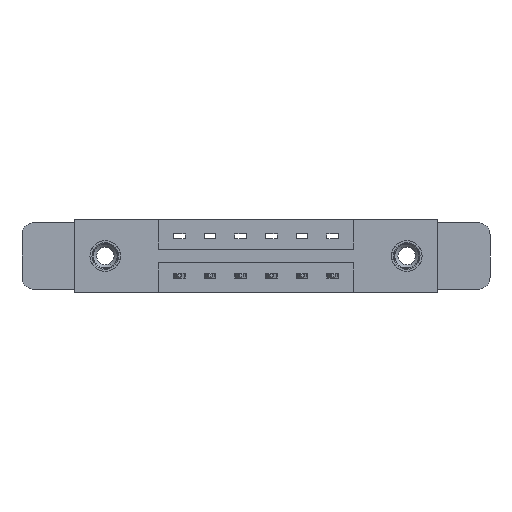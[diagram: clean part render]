
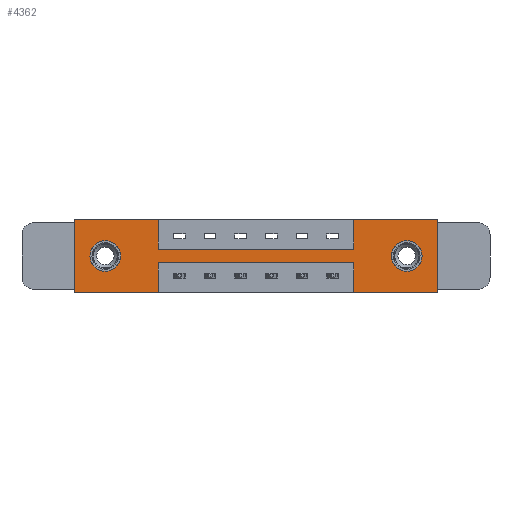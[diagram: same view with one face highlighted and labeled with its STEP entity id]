
A CAD part, front view. The second image highlights one B-rep face of the part: STEP entity #4362.
In plain terms, the highlighted planar face has unit normal (0, -1, 0).
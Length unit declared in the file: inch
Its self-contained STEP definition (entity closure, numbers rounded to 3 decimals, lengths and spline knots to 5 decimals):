
#9 = EDGE_LOOP ( 'NONE', ( #1963, #6554 ) ) ;
#53 = DIRECTION ( 'NONE',  ( 0., 1., 0. ) ) ;
#268 = VECTOR ( 'NONE', #10527, 39.37008 ) ;
#271 = VERTEX_POINT ( 'NONE', #1004 ) ;
#307 = DIRECTION ( 'NONE',  ( 0., 1., 0. ) ) ;
#468 = CARTESIAN_POINT ( 'NONE',  ( 0., 0., 0. ) ) ;
#487 = LINE ( 'NONE', #468, #2744 ) ;
#525 = CARTESIAN_POINT ( 'NONE',  ( 1.417, 0., -0.22 ) ) ;
#589 = DIRECTION ( 'NONE',  ( 0., -1., 0. ) ) ;
#739 = ORIENTED_EDGE ( 'NONE', *, *, #3154, .T. ) ;
#833 = EDGE_CURVE ( 'NONE', #2236, #11252, #10654, .T. ) ;
#843 = VERTEX_POINT ( 'NONE', #4582 ) ;
#922 = EDGE_CURVE ( 'NONE', #6024, #10262, #3065, .T. ) ;
#923 = VERTEX_POINT ( 'NONE', #1843 ) ;
#1004 = CARTESIAN_POINT ( 'NONE',  ( 0.425, 0., -0.15 ) ) ;
#1042 = CARTESIAN_POINT ( 'NONE',  ( 0.155, 0., -0.185 ) ) ;
#1116 = EDGE_CURVE ( 'NONE', #10430, #5213, #7602, .T. ) ;
#1382 = CARTESIAN_POINT ( 'NONE',  ( 0.425, 0., 0. ) ) ;
#1463 = LINE ( 'NONE', #9591, #10608 ) ;
#1606 = CARTESIAN_POINT ( 'NONE',  ( 0., 0., 0. ) ) ;
#1753 = CARTESIAN_POINT ( 'NONE',  ( 0., 0., -0.37 ) ) ;
#1778 = ORIENTED_EDGE ( 'NONE', *, *, #9428, .F. ) ;
#1800 = EDGE_CURVE ( 'NONE', #6470, #8813, #2345, .T. ) ;
#1843 = CARTESIAN_POINT ( 'NONE',  ( 0., 0., 0. ) ) ;
#1890 = EDGE_CURVE ( 'NONE', #10592, #6024, #8596, .T. ) ;
#1942 = DIRECTION ( 'NONE',  ( 0., 1., 0. ) ) ;
#1943 = DIRECTION ( 'NONE',  ( -1., 0., 0. ) ) ;
#1963 = ORIENTED_EDGE ( 'NONE', *, *, #833, .T. ) ;
#2064 = EDGE_LOOP ( 'NONE', ( #2796, #8260, #10268, #7159, #7033, #7247, #11724, #1778, #2246, #2922, #5707, #10975 ) ) ;
#2178 = CARTESIAN_POINT ( 'NONE',  ( 1.417, 0., 0. ) ) ;
#2236 = VERTEX_POINT ( 'NONE', #5588 ) ;
#2246 = ORIENTED_EDGE ( 'NONE', *, *, #11702, .F. ) ;
#2331 = CARTESIAN_POINT ( 'NONE',  ( 0., 0., -0.37 ) ) ;
#2345 = LINE ( 'NONE', #6467, #4595 ) ;
#2382 = LINE ( 'NONE', #1382, #268 ) ;
#2586 = EDGE_CURVE ( 'NONE', #10262, #6470, #1463, .T. ) ;
#2744 = VECTOR ( 'NONE', #6801, 39.37008 ) ;
#2754 = FACE_BOUND ( 'NONE', #9518, .T. ) ;
#2796 = ORIENTED_EDGE ( 'NONE', *, *, #2586, .F. ) ;
#2803 = CARTESIAN_POINT ( 'NONE',  ( 0.425, 0., -0.22 ) ) ;
#2817 = VECTOR ( 'NONE', #6248, 39.37008 ) ;
#2922 = ORIENTED_EDGE ( 'NONE', *, *, #11115, .F. ) ;
#3005 = VERTEX_POINT ( 'NONE', #10328 ) ;
#3065 = LINE ( 'NONE', #9972, #4051 ) ;
#3154 = EDGE_CURVE ( 'NONE', #843, #7137, #9260, .T. ) ;
#3186 = DIRECTION ( 'NONE',  ( 0., 0., 1. ) ) ;
#3655 = DIRECTION ( 'NONE',  ( 0., 0., 1. ) ) ;
#4051 = VECTOR ( 'NONE', #4507, 39.37008 ) ;
#4255 = LINE ( 'NONE', #5700, #9387 ) ;
#4362 = ADVANCED_FACE ( 'NONE', ( #5420, #2754, #9440 ), #5105, .T. ) ;
#4507 = DIRECTION ( 'NONE',  ( -1., 0., 0. ) ) ;
#4548 = CARTESIAN_POINT ( 'NONE',  ( 1.687, 0., -0.185 ) ) ;
#4582 = CARTESIAN_POINT ( 'NONE',  ( 0.155, 0., -0.107 ) ) ;
#4595 = VECTOR ( 'NONE', #1943, 39.37008 ) ;
#4645 = LINE ( 'NONE', #5330, #2817 ) ;
#4797 = VECTOR ( 'NONE', #9474, 39.37008 ) ;
#4827 = EDGE_CURVE ( 'NONE', #5213, #3005, #487, .T. ) ;
#4835 = DIRECTION ( 'NONE',  ( 0., 0., -1. ) ) ;
#4852 = AXIS2_PLACEMENT_3D ( 'NONE', #5870, #8636, #3186 ) ;
#5105 = PLANE ( 'NONE',  #8727 ) ;
#5134 = DIRECTION ( 'NONE',  ( 0., 0., -1. ) ) ;
#5213 = VERTEX_POINT ( 'NONE', #6055 ) ;
#5268 = AXIS2_PLACEMENT_3D ( 'NONE', #1042, #1942, #3655 ) ;
#5330 = CARTESIAN_POINT ( 'NONE',  ( 0., 0., -0.37 ) ) ;
#5352 = EDGE_CURVE ( 'NONE', #8813, #923, #8725, .T. ) ;
#5420 = FACE_BOUND ( 'NONE', #9, .T. ) ;
#5453 = AXIS2_PLACEMENT_3D ( 'NONE', #4548, #53, #5476 ) ;
#5476 = DIRECTION ( 'NONE',  ( 0., 0., -1. ) ) ;
#5588 = CARTESIAN_POINT ( 'NONE',  ( 1.687, 0., -0.107 ) ) ;
#5700 = CARTESIAN_POINT ( 'NONE',  ( 1.842, 0., 0. ) ) ;
#5707 = ORIENTED_EDGE ( 'NONE', *, *, #5352, .F. ) ;
#5870 = CARTESIAN_POINT ( 'NONE',  ( 0.155, 0., -0.185 ) ) ;
#6024 = VERTEX_POINT ( 'NONE', #525 ) ;
#6029 = CARTESIAN_POINT ( 'NONE',  ( 0.425, 0., 0. ) ) ;
#6055 = CARTESIAN_POINT ( 'NONE',  ( 1.417, 0., 0. ) ) ;
#6162 = VECTOR ( 'NONE', #7579, 39.37008 ) ;
#6248 = DIRECTION ( 'NONE',  ( -1., 0., 0. ) ) ;
#6366 = CARTESIAN_POINT ( 'NONE',  ( 1.417, 0., -0.37 ) ) ;
#6467 = CARTESIAN_POINT ( 'NONE',  ( 0., 0., -0.37 ) ) ;
#6470 = VERTEX_POINT ( 'NONE', #10317 ) ;
#6524 = CIRCLE ( 'NONE', #9713, 0.078 ) ;
#6554 = ORIENTED_EDGE ( 'NONE', *, *, #7571, .T. ) ;
#6642 = DIRECTION ( 'NONE',  ( 0., 0., -1. ) ) ;
#6801 = DIRECTION ( 'NONE',  ( 1., 0., 0. ) ) ;
#7033 = ORIENTED_EDGE ( 'NONE', *, *, #10008, .F. ) ;
#7137 = VERTEX_POINT ( 'NONE', #8942 ) ;
#7159 = ORIENTED_EDGE ( 'NONE', *, *, #8118, .F. ) ;
#7247 = ORIENTED_EDGE ( 'NONE', *, *, #4827, .F. ) ;
#7571 = EDGE_CURVE ( 'NONE', #11252, #2236, #6524, .T. ) ;
#7579 = DIRECTION ( 'NONE',  ( 0., 0., 1. ) ) ;
#7602 = LINE ( 'NONE', #2178, #8315 ) ;
#7781 = VERTEX_POINT ( 'NONE', #7788 ) ;
#7788 = CARTESIAN_POINT ( 'NONE',  ( 1.842, 0., -0.37 ) ) ;
#7966 = DIRECTION ( 'NONE',  ( 0., 0., 1. ) ) ;
#8118 = EDGE_CURVE ( 'NONE', #7781, #10592, #4645, .T. ) ;
#8260 = ORIENTED_EDGE ( 'NONE', *, *, #922, .F. ) ;
#8315 = VECTOR ( 'NONE', #11416, 39.37008 ) ;
#8461 = CARTESIAN_POINT ( 'NONE',  ( 0.425, 0., -0.15 ) ) ;
#8596 = LINE ( 'NONE', #11273, #6162 ) ;
#8601 = CARTESIAN_POINT ( 'NONE',  ( 0., 0., 0. ) ) ;
#8636 = DIRECTION ( 'NONE',  ( 0., 1., 0. ) ) ;
#8725 = LINE ( 'NONE', #1606, #10599 ) ;
#8726 = DIRECTION ( 'NONE',  ( 0., 0., -1. ) ) ;
#8727 = AXIS2_PLACEMENT_3D ( 'NONE', #2331, #589, #5134 ) ;
#8813 = VERTEX_POINT ( 'NONE', #1753 ) ;
#8942 = CARTESIAN_POINT ( 'NONE',  ( 0.155, 0., -0.263 ) ) ;
#9050 = EDGE_CURVE ( 'NONE', #7137, #843, #10054, .T. ) ;
#9260 = CIRCLE ( 'NONE', #5268, 0.078 ) ;
#9298 = ORIENTED_EDGE ( 'NONE', *, *, #9050, .T. ) ;
#9387 = VECTOR ( 'NONE', #4835, 39.37008 ) ;
#9428 = EDGE_CURVE ( 'NONE', #271, #10430, #11630, .T. ) ;
#9440 = FACE_OUTER_BOUND ( 'NONE', #2064, .T. ) ;
#9473 = VECTOR ( 'NONE', #10448, 39.37008 ) ;
#9474 = DIRECTION ( 'NONE',  ( 1., 0., 0. ) ) ;
#9518 = EDGE_LOOP ( 'NONE', ( #739, #9298 ) ) ;
#9591 = CARTESIAN_POINT ( 'NONE',  ( 0.425, 0., -0.37 ) ) ;
#9713 = AXIS2_PLACEMENT_3D ( 'NONE', #10417, #307, #6642 ) ;
#9972 = CARTESIAN_POINT ( 'NONE',  ( 0.425, 0., -0.22 ) ) ;
#10008 = EDGE_CURVE ( 'NONE', #3005, #7781, #4255, .T. ) ;
#10020 = VERTEX_POINT ( 'NONE', #6029 ) ;
#10054 = CIRCLE ( 'NONE', #4852, 0.078 ) ;
#10262 = VERTEX_POINT ( 'NONE', #2803 ) ;
#10268 = ORIENTED_EDGE ( 'NONE', *, *, #1890, .F. ) ;
#10301 = CARTESIAN_POINT ( 'NONE',  ( 1.417, 0., -0.15 ) ) ;
#10317 = CARTESIAN_POINT ( 'NONE',  ( 0.425, 0., -0.37 ) ) ;
#10328 = CARTESIAN_POINT ( 'NONE',  ( 1.842, 0., 0. ) ) ;
#10417 = CARTESIAN_POINT ( 'NONE',  ( 1.687, 0., -0.185 ) ) ;
#10430 = VERTEX_POINT ( 'NONE', #10301 ) ;
#10448 = DIRECTION ( 'NONE',  ( 1., 0., 0. ) ) ;
#10527 = DIRECTION ( 'NONE',  ( 0., 0., -1. ) ) ;
#10592 = VERTEX_POINT ( 'NONE', #6366 ) ;
#10599 = VECTOR ( 'NONE', #7966, 39.37008 ) ;
#10608 = VECTOR ( 'NONE', #8726, 39.37008 ) ;
#10654 = CIRCLE ( 'NONE', #5453, 0.078 ) ;
#10811 = CARTESIAN_POINT ( 'NONE',  ( 1.687, 0., -0.263 ) ) ;
#10975 = ORIENTED_EDGE ( 'NONE', *, *, #1800, .F. ) ;
#11115 = EDGE_CURVE ( 'NONE', #923, #10020, #11513, .T. ) ;
#11252 = VERTEX_POINT ( 'NONE', #10811 ) ;
#11273 = CARTESIAN_POINT ( 'NONE',  ( 1.417, 0., -0.37 ) ) ;
#11416 = DIRECTION ( 'NONE',  ( 0., 0., 1. ) ) ;
#11513 = LINE ( 'NONE', #8601, #4797 ) ;
#11630 = LINE ( 'NONE', #8461, #9473 ) ;
#11702 = EDGE_CURVE ( 'NONE', #10020, #271, #2382, .T. ) ;
#11724 = ORIENTED_EDGE ( 'NONE', *, *, #1116, .F. ) ;
